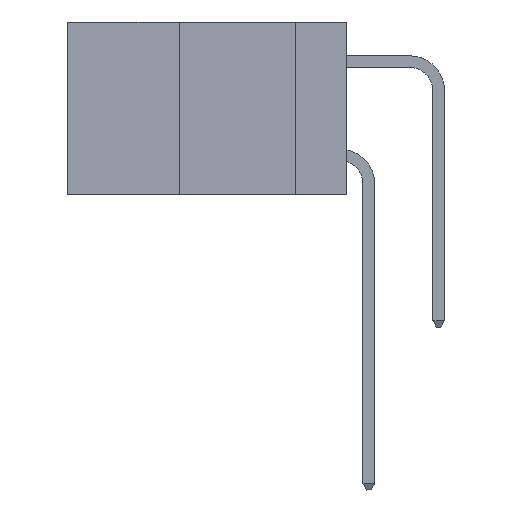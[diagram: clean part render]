
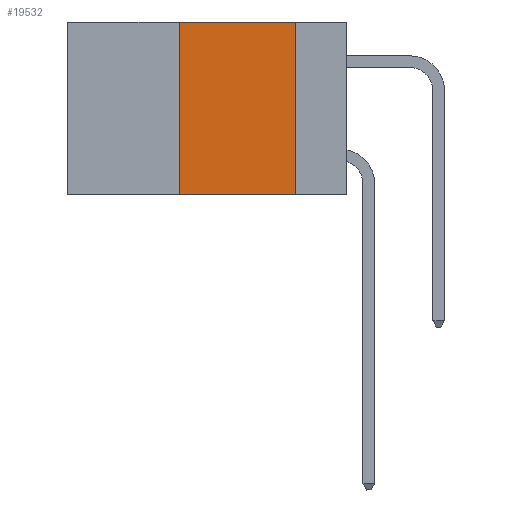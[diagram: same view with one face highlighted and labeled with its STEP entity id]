
A CAD part, left-side view. The second image highlights one B-rep face of the part: STEP entity #19532.
In plain terms, the highlighted planar face has unit normal (-1, 0, 0).
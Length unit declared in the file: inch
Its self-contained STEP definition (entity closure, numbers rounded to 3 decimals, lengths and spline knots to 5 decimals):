
#805 = PLANE ( 'NONE',  #21965 ) ;
#1037 = VECTOR ( 'NONE', #21784, 39.37008 ) ;
#2401 = VECTOR ( 'NONE', #21468, 39.37008 ) ;
#3002 = ORIENTED_EDGE ( 'NONE', *, *, #11860, .F. ) ;
#3386 = CARTESIAN_POINT ( 'NONE',  ( 0., 0.11, -0.37 ) ) ;
#3446 = LINE ( 'NONE', #9061, #4251 ) ;
#4251 = VECTOR ( 'NONE', #11160, 39.37008 ) ;
#4368 = VERTEX_POINT ( 'NONE', #20501 ) ;
#4657 = ORIENTED_EDGE ( 'NONE', *, *, #23047, .T. ) ;
#5563 = EDGE_CURVE ( 'NONE', #4368, #13073, #3446, .T. ) ;
#6087 = DIRECTION ( 'NONE',  ( 1., 0., 0. ) ) ;
#7905 = VECTOR ( 'NONE', #8979, 39.37008 ) ;
#7933 = FACE_OUTER_BOUND ( 'NONE', #15379, .T. ) ;
#8753 = LINE ( 'NONE', #20329, #7905 ) ;
#8979 = DIRECTION ( 'NONE',  ( 0., -1., 0. ) ) ;
#9061 = CARTESIAN_POINT ( 'NONE',  ( 0., 0.36, 0. ) ) ;
#10052 = ORIENTED_EDGE ( 'NONE', *, *, #13565, .F. ) ;
#10568 = CARTESIAN_POINT ( 'NONE',  ( 0., 0.6, -0.37 ) ) ;
#11160 = DIRECTION ( 'NONE',  ( 0., 0., 1. ) ) ;
#11860 = EDGE_CURVE ( 'NONE', #21663, #13349, #16210, .T. ) ;
#13073 = VERTEX_POINT ( 'NONE', #13800 ) ;
#13349 = VERTEX_POINT ( 'NONE', #3386 ) ;
#13565 = EDGE_CURVE ( 'NONE', #13073, #21663, #8753, .T. ) ;
#13800 = CARTESIAN_POINT ( 'NONE',  ( 0., 0.36, 0. ) ) ;
#15182 = CARTESIAN_POINT ( 'NONE',  ( 0., 0.11, 0. ) ) ;
#15379 = EDGE_LOOP ( 'NONE', ( #3002, #10052, #19377, #4657 ) ) ;
#16210 = LINE ( 'NONE', #17685, #2401 ) ;
#17533 = DIRECTION ( 'NONE',  ( 0., 0., -1. ) ) ;
#17685 = CARTESIAN_POINT ( 'NONE',  ( 0., 0.11, 0. ) ) ;
#17883 = LINE ( 'NONE', #10568, #1037 ) ;
#19377 = ORIENTED_EDGE ( 'NONE', *, *, #5563, .F. ) ;
#19532 = ADVANCED_FACE ( 'NONE', ( #7933 ), #805, .F. ) ;
#20329 = CARTESIAN_POINT ( 'NONE',  ( 0., 0.6, 0. ) ) ;
#20501 = CARTESIAN_POINT ( 'NONE',  ( 0., 0.36, -0.37 ) ) ;
#21085 = CARTESIAN_POINT ( 'NONE',  ( 0., 0.6, 0. ) ) ;
#21468 = DIRECTION ( 'NONE',  ( 0., 0., -1. ) ) ;
#21663 = VERTEX_POINT ( 'NONE', #15182 ) ;
#21784 = DIRECTION ( 'NONE',  ( 0., -1., 0. ) ) ;
#21965 = AXIS2_PLACEMENT_3D ( 'NONE', #21085, #6087, #17533 ) ;
#23047 = EDGE_CURVE ( 'NONE', #4368, #13349, #17883, .T. ) ;
